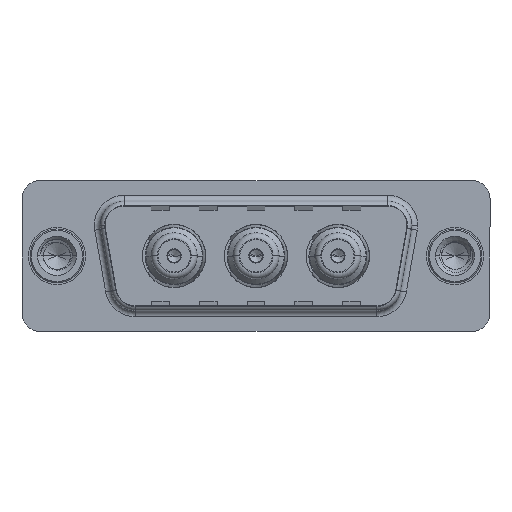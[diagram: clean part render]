
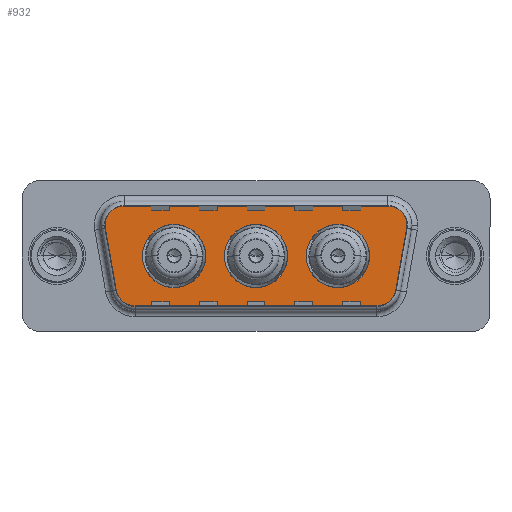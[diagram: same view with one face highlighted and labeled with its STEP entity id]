
A CAD part, top view. The second image highlights one B-rep face of the part: STEP entity #932.
In plain terms, the highlighted planar face has unit normal (0, 0, 1).
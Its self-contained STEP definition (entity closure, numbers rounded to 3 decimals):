
#259 = ORIENTED_EDGE ( 'NONE', *, *, #22400, .T. ) ;
#277 = CIRCLE ( 'NONE', #5386, 2.65 ) ;
#393 = CARTESIAN_POINT ( 'NONE',  ( 27.889, 4.9, 0. ) ) ;
#398 = DIRECTION ( 'NONE',  ( -1., 0., 0. ) ) ;
#560 = DIRECTION ( 'NONE',  ( 0., 0., 1. ) ) ;
#692 = CARTESIAN_POINT ( 'NONE',  ( 28.836, -3.247, 0. ) ) ;
#932 = ADVANCED_FACE ( 'NONE', ( #21043, #21584, #7214, #3156 ), #20518, .T. ) ;
#1137 = VECTOR ( 'NONE', #14409, 1000. ) ;
#1195 = VERTEX_POINT ( 'NONE', #21710 ) ;
#1246 = ORIENTED_EDGE ( 'NONE', *, *, #15863, .T. ) ;
#1637 = VERTEX_POINT ( 'NONE', #12282 ) ;
#1920 = VERTEX_POINT ( 'NONE', #11152 ) ;
#2178 = CIRCLE ( 'NONE', #7414, 2. ) ;
#2293 = CARTESIAN_POINT ( 'NONE',  ( 26.866, -2.9, 0. ) ) ;
#3156 = FACE_OUTER_BOUND ( 'NONE', #7657, .T. ) ;
#3283 = ORIENTED_EDGE ( 'NONE', *, *, #3839, .T. ) ;
#3400 = ORIENTED_EDGE ( 'NONE', *, *, #22462, .T. ) ;
#3444 = CARTESIAN_POINT ( 'NONE',  ( 12.45, 0., 0. ) ) ;
#3612 = VERTEX_POINT ( 'NONE', #7491 ) ;
#3839 = EDGE_CURVE ( 'NONE', #22160, #12532, #15089, .T. ) ;
#3866 = ORIENTED_EDGE ( 'NONE', *, *, #15446, .T. ) ;
#3943 = CARTESIAN_POINT ( 'NONE',  ( 9.8, 0., 0. ) ) ;
#4055 = DIRECTION ( 'NONE',  ( 1., 0., 0. ) ) ;
#4064 = AXIS2_PLACEMENT_3D ( 'NONE', #20348, #10024, #22090 ) ;
#4208 = DIRECTION ( 'NONE',  ( 0., 0., 1. ) ) ;
#4610 = CIRCLE ( 'NONE', #8786, 2.65 ) ;
#4828 = DIRECTION ( 'NONE',  ( 0., 0., 1. ) ) ;
#4885 = AXIS2_PLACEMENT_3D ( 'NONE', #20218, #9899, #21958 ) ;
#4917 = VECTOR ( 'NONE', #7228, 1000. ) ;
#4954 = VERTEX_POINT ( 'NONE', #22044 ) ;
#5054 = ORIENTED_EDGE ( 'NONE', *, *, #10421, .F. ) ;
#5281 = EDGE_LOOP ( 'NONE', ( #5689, #11739 ) ) ;
#5386 = AXIS2_PLACEMENT_3D ( 'NONE', #15295, #4828, #17008 ) ;
#5452 = EDGE_CURVE ( 'NONE', #16996, #3612, #9569, .T. ) ;
#5688 = DIRECTION ( 'NONE',  ( 1., 0., 0. ) ) ;
#5689 = ORIENTED_EDGE ( 'NONE', *, *, #18966, .F. ) ;
#6412 = AXIS2_PLACEMENT_3D ( 'NONE', #21216, #10898, #398 ) ;
#6635 = CARTESIAN_POINT ( 'NONE',  ( 5.411, 2.9, 0. ) ) ;
#6658 = CIRCLE ( 'NONE', #10731, 2. ) ;
#7153 = CARTESIAN_POINT ( 'NONE',  ( 3.441, 2.553, 0. ) ) ;
#7214 = FACE_BOUND ( 'NONE', #13487, .T. ) ;
#7228 = DIRECTION ( 'NONE',  ( 0.174, -0.985, 0. ) ) ;
#7414 = AXIS2_PLACEMENT_3D ( 'NONE', #11058, #560, #12804 ) ;
#7457 = ORIENTED_EDGE ( 'NONE', *, *, #17234, .T. ) ;
#7480 = CIRCLE ( 'NONE', #16143, 2.65 ) ;
#7491 = CARTESIAN_POINT ( 'NONE',  ( 4.464, -3.247, 0. ) ) ;
#7615 = VERTEX_POINT ( 'NONE', #19601 ) ;
#7619 = AXIS2_PLACEMENT_3D ( 'NONE', #19726, #20908, #20956 ) ;
#7632 = CIRCLE ( 'NONE', #9497, 2. ) ;
#7657 = EDGE_LOOP ( 'NONE', ( #3866, #3283, #7457, #259, #15678, #16409, #16256, #1246, #3400 ) ) ;
#8403 = DIRECTION ( 'NONE',  ( 1., 0., 0. ) ) ;
#8423 = CARTESIAN_POINT ( 'NONE',  ( 5.411, 4.9, 0. ) ) ;
#8574 = CARTESIAN_POINT ( 'NONE',  ( 5.411, 4.9, 0. ) ) ;
#8641 = LINE ( 'NONE', #8423, #21871 ) ;
#8786 = AXIS2_PLACEMENT_3D ( 'NONE', #3943, #16159, #5688 ) ;
#9301 = CARTESIAN_POINT ( 'NONE',  ( 29.889, 2.9, 0. ) ) ;
#9337 = EDGE_CURVE ( 'NONE', #16114, #16563, #8641, .T. ) ;
#9497 = AXIS2_PLACEMENT_3D ( 'NONE', #2293, #14553, #4055 ) ;
#9569 = LINE ( 'NONE', #7153, #4917 ) ;
#9639 = ORIENTED_EDGE ( 'NONE', *, *, #19561, .F. ) ;
#9773 = DIRECTION ( 'NONE',  ( 0., 0., 1. ) ) ;
#9800 = CIRCLE ( 'NONE', #6412, 2. ) ;
#9866 = VECTOR ( 'NONE', #18874, 1000. ) ;
#9899 = DIRECTION ( 'NONE',  ( 0., 0., 1. ) ) ;
#10024 = DIRECTION ( 'NONE',  ( 0., 0., 1. ) ) ;
#10092 = CARTESIAN_POINT ( 'NONE',  ( 23.5, 0., 0. ) ) ;
#10296 = CIRCLE ( 'NONE', #18675, 2.65 ) ;
#10421 = EDGE_CURVE ( 'NONE', #1195, #4954, #7480, .T. ) ;
#10731 = AXIS2_PLACEMENT_3D ( 'NONE', #6635, #18789, #8403 ) ;
#10898 = DIRECTION ( 'NONE',  ( 0., 0., 1. ) ) ;
#11058 = CARTESIAN_POINT ( 'NONE',  ( 6.434, -2.9, 0. ) ) ;
#11152 = CARTESIAN_POINT ( 'NONE',  ( 20.85, 0., 0. ) ) ;
#11352 = VERTEX_POINT ( 'NONE', #15998 ) ;
#11739 = ORIENTED_EDGE ( 'NONE', *, *, #18395, .F. ) ;
#11851 = DIRECTION ( 'NONE',  ( 1., 0., 0. ) ) ;
#11880 = CARTESIAN_POINT ( 'NONE',  ( 29.859, 2.553, 0. ) ) ;
#11940 = CARTESIAN_POINT ( 'NONE',  ( 6.434, -4.9, 0. ) ) ;
#12282 = CARTESIAN_POINT ( 'NONE',  ( 26.15, 0., 0. ) ) ;
#12532 = VERTEX_POINT ( 'NONE', #17213 ) ;
#12804 = DIRECTION ( 'NONE',  ( -1., 0., 0. ) ) ;
#13038 = EDGE_LOOP ( 'NONE', ( #21337, #5054 ) ) ;
#13487 = EDGE_LOOP ( 'NONE', ( #16837, #9639 ) ) ;
#14102 = VERTEX_POINT ( 'NONE', #3444 ) ;
#14409 = DIRECTION ( 'NONE',  ( 0.174, 0.985, 0. ) ) ;
#14532 = LINE ( 'NONE', #11940, #9866 ) ;
#14553 = DIRECTION ( 'NONE',  ( 0., 0., 1. ) ) ;
#14683 = CARTESIAN_POINT ( 'NONE',  ( 16.65, 0., 0. ) ) ;
#15089 = LINE ( 'NONE', #11880, #1137 ) ;
#15295 = CARTESIAN_POINT ( 'NONE',  ( 16.65, 0., 0. ) ) ;
#15446 = EDGE_CURVE ( 'NONE', #17122, #22160, #7632, .T. ) ;
#15515 = CARTESIAN_POINT ( 'NONE',  ( 3.441, 2.553, 0. ) ) ;
#15623 = CIRCLE ( 'NONE', #4064, 2. ) ;
#15678 = ORIENTED_EDGE ( 'NONE', *, *, #9337, .T. ) ;
#15863 = EDGE_CURVE ( 'NONE', #3612, #11352, #2178, .T. ) ;
#15871 = VERTEX_POINT ( 'NONE', #9301 ) ;
#15998 = CARTESIAN_POINT ( 'NONE',  ( 6.434, -4.9, 0. ) ) ;
#16114 = VERTEX_POINT ( 'NONE', #393 ) ;
#16143 = AXIS2_PLACEMENT_3D ( 'NONE', #14683, #4208, #16392 ) ;
#16159 = DIRECTION ( 'NONE',  ( 0., 0., 1. ) ) ;
#16256 = ORIENTED_EDGE ( 'NONE', *, *, #5452, .T. ) ;
#16392 = DIRECTION ( 'NONE',  ( 1., 0., 0. ) ) ;
#16409 = ORIENTED_EDGE ( 'NONE', *, *, #19642, .T. ) ;
#16490 = CIRCLE ( 'NONE', #4885, 2.65 ) ;
#16563 = VERTEX_POINT ( 'NONE', #8574 ) ;
#16837 = ORIENTED_EDGE ( 'NONE', *, *, #17239, .F. ) ;
#16996 = VERTEX_POINT ( 'NONE', #15515 ) ;
#17008 = DIRECTION ( 'NONE',  ( 1., 0., 0. ) ) ;
#17122 = VERTEX_POINT ( 'NONE', #19220 ) ;
#17213 = CARTESIAN_POINT ( 'NONE',  ( 29.859, 2.553, 0. ) ) ;
#17234 = EDGE_CURVE ( 'NONE', #12532, #15871, #9800, .T. ) ;
#17239 = EDGE_CURVE ( 'NONE', #14102, #7615, #4610, .T. ) ;
#18395 = EDGE_CURVE ( 'NONE', #1920, #1637, #10296, .T. ) ;
#18675 = AXIS2_PLACEMENT_3D ( 'NONE', #10092, #22163, #11851 ) ;
#18789 = DIRECTION ( 'NONE',  ( 0., 0., 1. ) ) ;
#18874 = DIRECTION ( 'NONE',  ( 1., 0., 0. ) ) ;
#18966 = EDGE_CURVE ( 'NONE', #1637, #1920, #20498, .T. ) ;
#19220 = CARTESIAN_POINT ( 'NONE',  ( 26.866, -4.9, 0. ) ) ;
#19561 = EDGE_CURVE ( 'NONE', #7615, #14102, #16490, .T. ) ;
#19601 = CARTESIAN_POINT ( 'NONE',  ( 7.15, 0., 0. ) ) ;
#19642 = EDGE_CURVE ( 'NONE', #16563, #16996, #6658, .T. ) ;
#19726 = CARTESIAN_POINT ( 'NONE',  ( 26.866, -2.9, 0. ) ) ;
#20095 = CARTESIAN_POINT ( 'NONE',  ( 23.5, 0., 0. ) ) ;
#20218 = CARTESIAN_POINT ( 'NONE',  ( 9.8, 0., 0. ) ) ;
#20348 = CARTESIAN_POINT ( 'NONE',  ( 27.889, 2.9, 0. ) ) ;
#20498 = CIRCLE ( 'NONE', #22427, 2.65 ) ;
#20512 = DIRECTION ( 'NONE',  ( -1., 0., 0. ) ) ;
#20518 = PLANE ( 'NONE',  #7619 ) ;
#20908 = DIRECTION ( 'NONE',  ( 0., 0., 1. ) ) ;
#20956 = DIRECTION ( 'NONE',  ( 1., 0., 0. ) ) ;
#21043 = FACE_BOUND ( 'NONE', #13038, .T. ) ;
#21216 = CARTESIAN_POINT ( 'NONE',  ( 27.889, 2.9, 0. ) ) ;
#21337 = ORIENTED_EDGE ( 'NONE', *, *, #21543, .F. ) ;
#21543 = EDGE_CURVE ( 'NONE', #4954, #1195, #277, .T. ) ;
#21584 = FACE_BOUND ( 'NONE', #5281, .T. ) ;
#21710 = CARTESIAN_POINT ( 'NONE',  ( 14., 0., 0. ) ) ;
#21823 = DIRECTION ( 'NONE',  ( 1., 0., 0. ) ) ;
#21871 = VECTOR ( 'NONE', #20512, 1000. ) ;
#21958 = DIRECTION ( 'NONE',  ( 1., 0., 0. ) ) ;
#22044 = CARTESIAN_POINT ( 'NONE',  ( 19.3, 0., 0. ) ) ;
#22090 = DIRECTION ( 'NONE',  ( -1., 0., 0. ) ) ;
#22160 = VERTEX_POINT ( 'NONE', #692 ) ;
#22163 = DIRECTION ( 'NONE',  ( 0., 0., 1. ) ) ;
#22400 = EDGE_CURVE ( 'NONE', #15871, #16114, #15623, .T. ) ;
#22427 = AXIS2_PLACEMENT_3D ( 'NONE', #20095, #9773, #21823 ) ;
#22462 = EDGE_CURVE ( 'NONE', #11352, #17122, #14532, .T. ) ;
